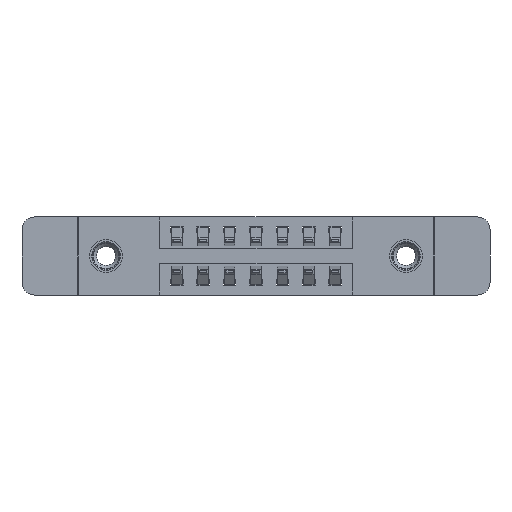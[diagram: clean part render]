
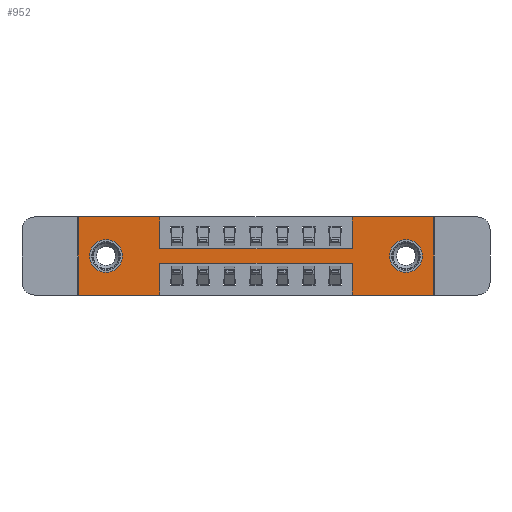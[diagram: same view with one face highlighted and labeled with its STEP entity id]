
A CAD part, front view. The second image highlights one B-rep face of the part: STEP entity #952.
In plain terms, the highlighted planar face has unit normal (0, -1, 0).
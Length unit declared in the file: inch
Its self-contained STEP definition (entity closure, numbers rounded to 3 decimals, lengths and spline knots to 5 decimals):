
#58 = DIRECTION ( 'NONE',  ( 1., 0., 0. ) ) ;
#687 = VERTEX_POINT ( 'NONE', #13858 ) ;
#697 = VERTEX_POINT ( 'NONE', #3337 ) ;
#783 = EDGE_LOOP ( 'NONE', ( #7142, #6881 ) ) ;
#918 = DIRECTION ( 'NONE',  ( 1., 0., 0. ) ) ;
#952 = ADVANCED_FACE ( 'NONE', ( #11654, #3317, #11360 ), #3396, .T. ) ;
#980 = CARTESIAN_POINT ( 'NONE',  ( 1.5525, 0., -0.263 ) ) ;
#1155 = LINE ( 'NONE', #3756, #10089 ) ;
#1255 = LINE ( 'NONE', #1475, #2417 ) ;
#1335 = VECTOR ( 'NONE', #58, 39.37008 ) ;
#1386 = CARTESIAN_POINT ( 'NONE',  ( 0.3875, 0., -0.22 ) ) ;
#1389 = VECTOR ( 'NONE', #7458, 39.37008 ) ;
#1393 = EDGE_CURVE ( 'NONE', #7303, #11986, #10765, .T. ) ;
#1475 = CARTESIAN_POINT ( 'NONE',  ( 0., 0., -0.37 ) ) ;
#1824 = AXIS2_PLACEMENT_3D ( 'NONE', #6319, #12090, #14339 ) ;
#2163 = CARTESIAN_POINT ( 'NONE',  ( 1.2975, 0., -0.37 ) ) ;
#2196 = ORIENTED_EDGE ( 'NONE', *, *, #12562, .F. ) ;
#2417 = VECTOR ( 'NONE', #10731, 39.37008 ) ;
#2419 = VERTEX_POINT ( 'NONE', #10724 ) ;
#2440 = ORIENTED_EDGE ( 'NONE', *, *, #5811, .F. ) ;
#2454 = CARTESIAN_POINT ( 'NONE',  ( 0.1325, 0., -0.185 ) ) ;
#2739 = DIRECTION ( 'NONE',  ( 0., 0., 1. ) ) ;
#2753 = CARTESIAN_POINT ( 'NONE',  ( 0.1325, 0., -0.185 ) ) ;
#3099 = EDGE_CURVE ( 'NONE', #13364, #8170, #9205, .T. ) ;
#3198 = ORIENTED_EDGE ( 'NONE', *, *, #10166, .F. ) ;
#3317 = FACE_BOUND ( 'NONE', #5843, .T. ) ;
#3337 = CARTESIAN_POINT ( 'NONE',  ( 1.2975, 0., -0.15 ) ) ;
#3396 = PLANE ( 'NONE',  #3512 ) ;
#3512 = AXIS2_PLACEMENT_3D ( 'NONE', #12650, #6811, #10366 ) ;
#3683 = VERTEX_POINT ( 'NONE', #4979 ) ;
#3756 = CARTESIAN_POINT ( 'NONE',  ( 1.2975, 0., 0. ) ) ;
#3764 = VECTOR ( 'NONE', #10425, 39.37008 ) ;
#3813 = ORIENTED_EDGE ( 'NONE', *, *, #7047, .T. ) ;
#3856 = EDGE_CURVE ( 'NONE', #10172, #11469, #12711, .T. ) ;
#3863 = VECTOR ( 'NONE', #7265, 39.37008 ) ;
#4292 = CARTESIAN_POINT ( 'NONE',  ( 1.685, 0., -0.37 ) ) ;
#4451 = EDGE_CURVE ( 'NONE', #11986, #7303, #9333, .T. ) ;
#4710 = LINE ( 'NONE', #11758, #1335 ) ;
#4782 = VECTOR ( 'NONE', #13708, 39.37008 ) ;
#4900 = CARTESIAN_POINT ( 'NONE',  ( 0., 0., 0. ) ) ;
#4912 = CARTESIAN_POINT ( 'NONE',  ( 0.3875, 0., -0.37 ) ) ;
#4949 = LINE ( 'NONE', #6022, #1389 ) ;
#4979 = CARTESIAN_POINT ( 'NONE',  ( 0., 0., 0. ) ) ;
#5022 = ORIENTED_EDGE ( 'NONE', *, *, #11429, .F. ) ;
#5285 = VERTEX_POINT ( 'NONE', #4292 ) ;
#5355 = CARTESIAN_POINT ( 'NONE',  ( 0.3875, 0., -0.15 ) ) ;
#5640 = DIRECTION ( 'NONE',  ( 0., 0., 1. ) ) ;
#5781 = DIRECTION ( 'NONE',  ( 0., 0., -1. ) ) ;
#5811 = EDGE_CURVE ( 'NONE', #697, #13364, #1155, .T. ) ;
#5843 = EDGE_LOOP ( 'NONE', ( #3813, #9453 ) ) ;
#5878 = VECTOR ( 'NONE', #918, 39.37008 ) ;
#6022 = CARTESIAN_POINT ( 'NONE',  ( 0., 0., -0.37 ) ) ;
#6319 = CARTESIAN_POINT ( 'NONE',  ( 1.5525, 0., -0.185 ) ) ;
#6499 = CIRCLE ( 'NONE', #10590, 0.078 ) ;
#6554 = DIRECTION ( 'NONE',  ( 0., 0., 1. ) ) ;
#6767 = CARTESIAN_POINT ( 'NONE',  ( 1.2975, 0., -0.37 ) ) ;
#6774 = ORIENTED_EDGE ( 'NONE', *, *, #3099, .F. ) ;
#6811 = DIRECTION ( 'NONE',  ( 0., -1., 0. ) ) ;
#6881 = ORIENTED_EDGE ( 'NONE', *, *, #4451, .T. ) ;
#7047 = EDGE_CURVE ( 'NONE', #8950, #2419, #6499, .T. ) ;
#7142 = ORIENTED_EDGE ( 'NONE', *, *, #1393, .T. ) ;
#7265 = DIRECTION ( 'NONE',  ( -1., 0., 0. ) ) ;
#7303 = VERTEX_POINT ( 'NONE', #14856 ) ;
#7304 = CARTESIAN_POINT ( 'NONE',  ( 0.1325, 0., -0.107 ) ) ;
#7306 = CARTESIAN_POINT ( 'NONE',  ( 0., 0., 0. ) ) ;
#7458 = DIRECTION ( 'NONE',  ( -1., 0., 0. ) ) ;
#7771 = CARTESIAN_POINT ( 'NONE',  ( 0., 0., 0. ) ) ;
#7942 = VECTOR ( 'NONE', #8925, 39.37008 ) ;
#8030 = LINE ( 'NONE', #12659, #3863 ) ;
#8123 = ORIENTED_EDGE ( 'NONE', *, *, #13392, .F. ) ;
#8170 = VERTEX_POINT ( 'NONE', #14760 ) ;
#8293 = DIRECTION ( 'NONE',  ( 0., 0., 1. ) ) ;
#8419 = AXIS2_PLACEMENT_3D ( 'NONE', #2753, #12021, #6554 ) ;
#8502 = LINE ( 'NONE', #7306, #13041 ) ;
#8508 = EDGE_CURVE ( 'NONE', #2419, #8950, #11095, .T. ) ;
#8515 = DIRECTION ( 'NONE',  ( 1., 0., 0. ) ) ;
#8876 = CARTESIAN_POINT ( 'NONE',  ( 1.2975, 0., -0.22 ) ) ;
#8925 = DIRECTION ( 'NONE',  ( 0., 0., -1. ) ) ;
#8950 = VERTEX_POINT ( 'NONE', #7304 ) ;
#9000 = CARTESIAN_POINT ( 'NONE',  ( 1.685, 0., 0. ) ) ;
#9035 = VERTEX_POINT ( 'NONE', #6767 ) ;
#9141 = CARTESIAN_POINT ( 'NONE',  ( 1.2975, 0., 0. ) ) ;
#9205 = LINE ( 'NONE', #7771, #5878 ) ;
#9290 = EDGE_CURVE ( 'NONE', #14707, #14031, #13414, .T. ) ;
#9333 = CIRCLE ( 'NONE', #1824, 0.078 ) ;
#9453 = ORIENTED_EDGE ( 'NONE', *, *, #8508, .T. ) ;
#9514 = DIRECTION ( 'NONE',  ( 0., 0., 1. ) ) ;
#9673 = VERTEX_POINT ( 'NONE', #8876 ) ;
#9895 = EDGE_CURVE ( 'NONE', #8170, #5285, #12268, .T. ) ;
#10089 = VECTOR ( 'NONE', #8293, 39.37008 ) ;
#10166 = EDGE_CURVE ( 'NONE', #3683, #14707, #14433, .T. ) ;
#10172 = VERTEX_POINT ( 'NONE', #1386 ) ;
#10366 = DIRECTION ( 'NONE',  ( 0., 0., -1. ) ) ;
#10425 = DIRECTION ( 'NONE',  ( 0., 0., -1. ) ) ;
#10568 = DIRECTION ( 'NONE',  ( 0., 1., 0. ) ) ;
#10590 = AXIS2_PLACEMENT_3D ( 'NONE', #2454, #10568, #9514 ) ;
#10674 = EDGE_CURVE ( 'NONE', #5285, #9035, #4949, .T. ) ;
#10724 = CARTESIAN_POINT ( 'NONE',  ( 0.1325, 0., -0.263 ) ) ;
#10725 = EDGE_CURVE ( 'NONE', #687, #3683, #8502, .T. ) ;
#10731 = DIRECTION ( 'NONE',  ( -1., 0., 0. ) ) ;
#10765 = CIRCLE ( 'NONE', #14196, 0.078 ) ;
#11095 = CIRCLE ( 'NONE', #8419, 0.078 ) ;
#11360 = FACE_OUTER_BOUND ( 'NONE', #13262, .T. ) ;
#11405 = ORIENTED_EDGE ( 'NONE', *, *, #14704, .F. ) ;
#11429 = EDGE_CURVE ( 'NONE', #9673, #10172, #8030, .T. ) ;
#11469 = VERTEX_POINT ( 'NONE', #4912 ) ;
#11621 = ORIENTED_EDGE ( 'NONE', *, *, #10674, .F. ) ;
#11654 = FACE_BOUND ( 'NONE', #783, .T. ) ;
#11684 = ORIENTED_EDGE ( 'NONE', *, *, #9290, .F. ) ;
#11758 = CARTESIAN_POINT ( 'NONE',  ( 0.3875, 0., -0.15 ) ) ;
#11833 = ORIENTED_EDGE ( 'NONE', *, *, #9895, .F. ) ;
#11986 = VERTEX_POINT ( 'NONE', #980 ) ;
#12021 = DIRECTION ( 'NONE',  ( 0., 1., 0. ) ) ;
#12025 = VECTOR ( 'NONE', #5640, 39.37008 ) ;
#12090 = DIRECTION ( 'NONE',  ( 0., 1., 0. ) ) ;
#12268 = LINE ( 'NONE', #9000, #7942 ) ;
#12390 = ORIENTED_EDGE ( 'NONE', *, *, #10725, .F. ) ;
#12470 = ORIENTED_EDGE ( 'NONE', *, *, #3856, .F. ) ;
#12562 = EDGE_CURVE ( 'NONE', #11469, #687, #1255, .T. ) ;
#12650 = CARTESIAN_POINT ( 'NONE',  ( 0., 0., -0.37 ) ) ;
#12659 = CARTESIAN_POINT ( 'NONE',  ( 0.3875, 0., -0.22 ) ) ;
#12686 = DIRECTION ( 'NONE',  ( 0., 1., 0. ) ) ;
#12711 = LINE ( 'NONE', #14747, #3764 ) ;
#12840 = CARTESIAN_POINT ( 'NONE',  ( 1.5525, 0., -0.185 ) ) ;
#13041 = VECTOR ( 'NONE', #2739, 39.37008 ) ;
#13262 = EDGE_LOOP ( 'NONE', ( #12470, #5022, #8123, #11621, #11833, #6774, #2440, #11405, #11684, #3198, #12390, #2196 ) ) ;
#13364 = VERTEX_POINT ( 'NONE', #9141 ) ;
#13392 = EDGE_CURVE ( 'NONE', #9035, #9673, #13678, .T. ) ;
#13414 = LINE ( 'NONE', #14608, #4782 ) ;
#13678 = LINE ( 'NONE', #2163, #12025 ) ;
#13708 = DIRECTION ( 'NONE',  ( 0., 0., -1. ) ) ;
#13858 = CARTESIAN_POINT ( 'NONE',  ( 0., 0., -0.37 ) ) ;
#13945 = CARTESIAN_POINT ( 'NONE',  ( 0.3875, 0., 0. ) ) ;
#14031 = VERTEX_POINT ( 'NONE', #5355 ) ;
#14196 = AXIS2_PLACEMENT_3D ( 'NONE', #12840, #12686, #5781 ) ;
#14339 = DIRECTION ( 'NONE',  ( 0., 0., -1. ) ) ;
#14433 = LINE ( 'NONE', #4900, #14946 ) ;
#14608 = CARTESIAN_POINT ( 'NONE',  ( 0.3875, 0., 0. ) ) ;
#14704 = EDGE_CURVE ( 'NONE', #14031, #697, #4710, .T. ) ;
#14707 = VERTEX_POINT ( 'NONE', #13945 ) ;
#14747 = CARTESIAN_POINT ( 'NONE',  ( 0.3875, 0., -0.37 ) ) ;
#14760 = CARTESIAN_POINT ( 'NONE',  ( 1.685, 0., 0. ) ) ;
#14856 = CARTESIAN_POINT ( 'NONE',  ( 1.5525, 0., -0.107 ) ) ;
#14946 = VECTOR ( 'NONE', #8515, 39.37008 ) ;
